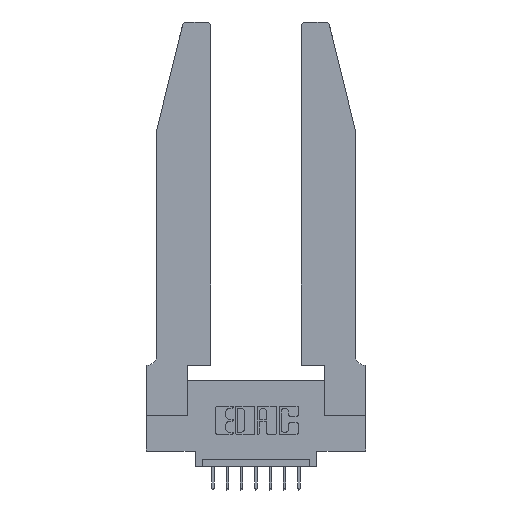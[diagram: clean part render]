
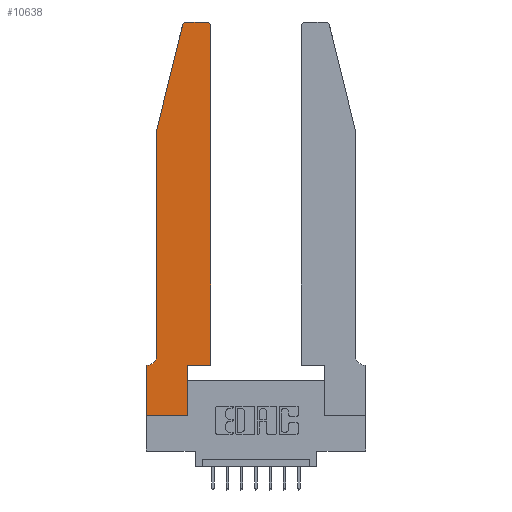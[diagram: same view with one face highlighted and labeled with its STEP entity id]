
A CAD part, top view. The second image highlights one B-rep face of the part: STEP entity #10638.
In plain terms, the highlighted planar face has unit normal (0, 0, 1).
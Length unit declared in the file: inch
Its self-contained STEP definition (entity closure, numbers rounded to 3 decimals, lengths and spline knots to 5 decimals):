
#165 = LINE ( 'NONE', #12544, #4356 ) ;
#270 = CARTESIAN_POINT ( 'NONE',  ( 0., 0., 0.37 ) ) ;
#394 = CARTESIAN_POINT ( 'NONE',  ( 0.4205, 2.72, 0.37 ) ) ;
#409 = CARTESIAN_POINT ( 'NONE',  ( 0.0755, 2., 0.37 ) ) ;
#593 = ORIENTED_EDGE ( 'NONE', *, *, #13928, .T. ) ;
#753 = LINE ( 'NONE', #409, #7079 ) ;
#1013 = PLANE ( 'NONE',  #12865 ) ;
#1020 = ORIENTED_EDGE ( 'NONE', *, *, #9072, .T. ) ;
#1021 = DIRECTION ( 'NONE',  ( 0., -1., 0. ) ) ;
#1079 = CIRCLE ( 'NONE', #7417, 0.07 ) ;
#1156 = EDGE_CURVE ( 'NONE', #8766, #4156, #1079, .T. ) ;
#1202 = EDGE_CURVE ( 'NONE', #4156, #3705, #7227, .T. ) ;
#1412 = EDGE_CURVE ( 'NONE', #13406, #1643, #13506, .T. ) ;
#1643 = VERTEX_POINT ( 'NONE', #5912 ) ;
#1737 = CARTESIAN_POINT ( 'NONE',  ( 0.284, 2.72, 0.37 ) ) ;
#1816 = CIRCLE ( 'NONE', #8678, 0.03 ) ;
#2016 = ORIENTED_EDGE ( 'NONE', *, *, #2851, .T. ) ;
#2068 = EDGE_CURVE ( 'NONE', #14697, #8766, #753, .T. ) ;
#2111 = AXIS2_PLACEMENT_3D ( 'NONE', #394, #8504, #14120 ) ;
#2186 = ORIENTED_EDGE ( 'NONE', *, *, #1156, .T. ) ;
#2519 = VERTEX_POINT ( 'NONE', #12879 ) ;
#2636 = CARTESIAN_POINT ( 'NONE',  ( 0.0755, 0.35, 0.37 ) ) ;
#2661 = EDGE_LOOP ( 'NONE', ( #593, #9741, #1020, #7549, #2186, #14928, #6354, #4169, #14814, #2016, #4570, #8235 ) ) ;
#2851 = EDGE_CURVE ( 'NONE', #10995, #13406, #14809, .T. ) ;
#3050 = EDGE_CURVE ( 'NONE', #6515, #4661, #1816, .T. ) ;
#3124 = CARTESIAN_POINT ( 'NONE',  ( 0.4505, 0.35, 0.37 ) ) ;
#3229 = CARTESIAN_POINT ( 'NONE',  ( 0.4505, 0.35, 0.37 ) ) ;
#3324 = CARTESIAN_POINT ( 'NONE',  ( 0.284, 2.75, 0.37 ) ) ;
#3705 = VERTEX_POINT ( 'NONE', #9253 ) ;
#3713 = CARTESIAN_POINT ( 'NONE',  ( 0.0755, 2., 0.37 ) ) ;
#3993 = EDGE_CURVE ( 'NONE', #1643, #2519, #11338, .T. ) ;
#4156 = VERTEX_POINT ( 'NONE', #5442 ) ;
#4169 = ORIENTED_EDGE ( 'NONE', *, *, #11396, .T. ) ;
#4304 = LINE ( 'NONE', #3713, #4843 ) ;
#4356 = VECTOR ( 'NONE', #5940, 39.37008 ) ;
#4364 = DIRECTION ( 'NONE',  ( 0., 0., 1. ) ) ;
#4570 = ORIENTED_EDGE ( 'NONE', *, *, #1412, .T. ) ;
#4661 = VERTEX_POINT ( 'NONE', #8987 ) ;
#4843 = VECTOR ( 'NONE', #7184, 39.37008 ) ;
#5442 = CARTESIAN_POINT ( 'NONE',  ( 0.0055, 0.35, 0.37 ) ) ;
#5607 = DIRECTION ( 'NONE',  ( 1., 0., 0. ) ) ;
#5912 = CARTESIAN_POINT ( 'NONE',  ( 0.4505, 2.72, 0.37 ) ) ;
#5940 = DIRECTION ( 'NONE',  ( -1., 0., 0. ) ) ;
#6155 = VECTOR ( 'NONE', #10701, 39.37008 ) ;
#6299 = VECTOR ( 'NONE', #10400, 39.37008 ) ;
#6354 = ORIENTED_EDGE ( 'NONE', *, *, #13879, .T. ) ;
#6515 = VERTEX_POINT ( 'NONE', #3324 ) ;
#7079 = VECTOR ( 'NONE', #14287, 39.37008 ) ;
#7184 = DIRECTION ( 'NONE',  ( -0.239, -0.971, 0. ) ) ;
#7227 = LINE ( 'NONE', #2636, #6155 ) ;
#7235 = DIRECTION ( 'NONE',  ( 0., 0., -1. ) ) ;
#7317 = VECTOR ( 'NONE', #11685, 39.37008 ) ;
#7410 = CARTESIAN_POINT ( 'NONE',  ( 0.2865, 0., 0.37 ) ) ;
#7417 = AXIS2_PLACEMENT_3D ( 'NONE', #12943, #7235, #9485 ) ;
#7549 = ORIENTED_EDGE ( 'NONE', *, *, #2068, .T. ) ;
#7647 = CARTESIAN_POINT ( 'NONE',  ( 0.4505, 0.35, 0.37 ) ) ;
#8133 = VECTOR ( 'NONE', #14616, 39.37008 ) ;
#8235 = ORIENTED_EDGE ( 'NONE', *, *, #3993, .T. ) ;
#8504 = DIRECTION ( 'NONE',  ( 0., 0., 1. ) ) ;
#8507 = LINE ( 'NONE', #14787, #12084 ) ;
#8652 = VERTEX_POINT ( 'NONE', #7410 ) ;
#8678 = AXIS2_PLACEMENT_3D ( 'NONE', #1737, #14178, #10812 ) ;
#8766 = VERTEX_POINT ( 'NONE', #13516 ) ;
#8926 = EDGE_CURVE ( 'NONE', #8652, #10995, #14385, .T. ) ;
#8987 = CARTESIAN_POINT ( 'NONE',  ( 0.25487, 2.72718, 0.37 ) ) ;
#9072 = EDGE_CURVE ( 'NONE', #4661, #14697, #4304, .T. ) ;
#9253 = CARTESIAN_POINT ( 'NONE',  ( 0., 0.35, 0.37 ) ) ;
#9485 = DIRECTION ( 'NONE',  ( -1., 0., 0. ) ) ;
#9741 = ORIENTED_EDGE ( 'NONE', *, *, #3050, .T. ) ;
#10400 = DIRECTION ( 'NONE',  ( 0., 1., 0. ) ) ;
#10491 = CARTESIAN_POINT ( 'NONE',  ( 0.0755, 2., 0.37 ) ) ;
#10638 = ADVANCED_FACE ( 'NONE', ( #12893 ), #1013, .T. ) ;
#10642 = CARTESIAN_POINT ( 'NONE',  ( 0.2865, 0.35, 0.37 ) ) ;
#10701 = DIRECTION ( 'NONE',  ( -1., 0., 0. ) ) ;
#10812 = DIRECTION ( 'NONE',  ( 1., 0., 0. ) ) ;
#10952 = VERTEX_POINT ( 'NONE', #270 ) ;
#10995 = VERTEX_POINT ( 'NONE', #10642 ) ;
#11338 = CIRCLE ( 'NONE', #2111, 0.03 ) ;
#11396 = EDGE_CURVE ( 'NONE', #10952, #8652, #12340, .T. ) ;
#11454 = CARTESIAN_POINT ( 'NONE',  ( 0.2865, 0.35, 0.37 ) ) ;
#11685 = DIRECTION ( 'NONE',  ( 1., 0., 0. ) ) ;
#12084 = VECTOR ( 'NONE', #1021, 39.37008 ) ;
#12340 = LINE ( 'NONE', #12813, #7317 ) ;
#12544 = CARTESIAN_POINT ( 'NONE',  ( 0.2605, 2.75, 0.37 ) ) ;
#12813 = CARTESIAN_POINT ( 'NONE',  ( 0., 0., 0.37 ) ) ;
#12865 = AXIS2_PLACEMENT_3D ( 'NONE', #14877, #4364, #13700 ) ;
#12879 = CARTESIAN_POINT ( 'NONE',  ( 0.4205, 2.75, 0.37 ) ) ;
#12893 = FACE_OUTER_BOUND ( 'NONE', #2661, .T. ) ;
#12943 = CARTESIAN_POINT ( 'NONE',  ( 0.0055, 0.42, 0.37 ) ) ;
#13406 = VERTEX_POINT ( 'NONE', #3229 ) ;
#13506 = LINE ( 'NONE', #7647, #8133 ) ;
#13516 = CARTESIAN_POINT ( 'NONE',  ( 0.0755, 0.42, 0.37 ) ) ;
#13700 = DIRECTION ( 'NONE',  ( 1., 0., 0. ) ) ;
#13879 = EDGE_CURVE ( 'NONE', #3705, #10952, #8507, .T. ) ;
#13928 = EDGE_CURVE ( 'NONE', #2519, #6515, #165, .T. ) ;
#14072 = VECTOR ( 'NONE', #5607, 39.37008 ) ;
#14120 = DIRECTION ( 'NONE',  ( 1., 0., 0. ) ) ;
#14178 = DIRECTION ( 'NONE',  ( 0., 0., 1. ) ) ;
#14287 = DIRECTION ( 'NONE',  ( 0., -1., 0. ) ) ;
#14385 = LINE ( 'NONE', #11454, #6299 ) ;
#14616 = DIRECTION ( 'NONE',  ( 0., 1., 0. ) ) ;
#14697 = VERTEX_POINT ( 'NONE', #10491 ) ;
#14787 = CARTESIAN_POINT ( 'NONE',  ( 0., 0., 0.37 ) ) ;
#14809 = LINE ( 'NONE', #3124, #14072 ) ;
#14814 = ORIENTED_EDGE ( 'NONE', *, *, #8926, .T. ) ;
#14877 = CARTESIAN_POINT ( 'NONE',  ( 0., 0.35, 0.37 ) ) ;
#14928 = ORIENTED_EDGE ( 'NONE', *, *, #1202, .T. ) ;
